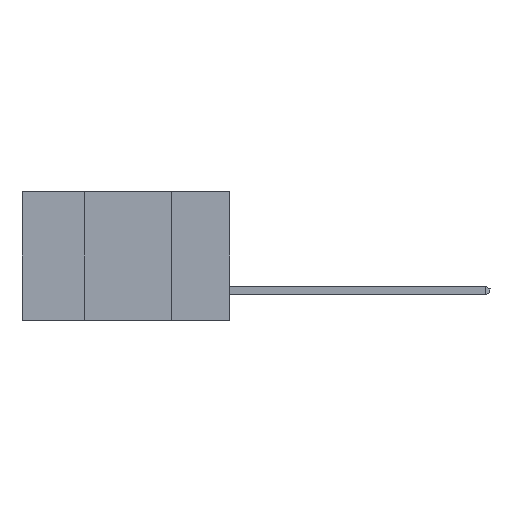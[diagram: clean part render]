
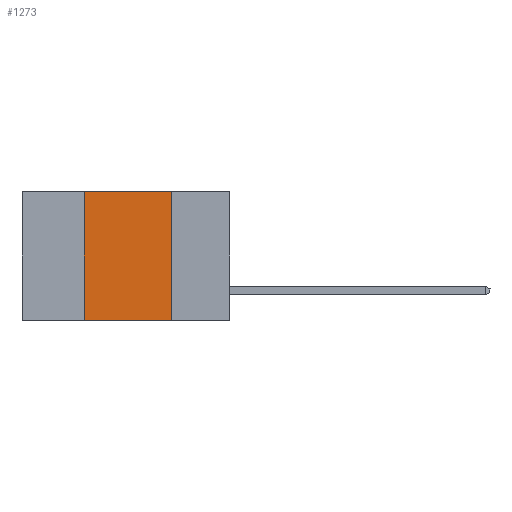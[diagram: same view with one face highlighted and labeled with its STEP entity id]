
A CAD part, left-side view. The second image highlights one B-rep face of the part: STEP entity #1273.
In plain terms, the highlighted planar face has unit normal (-1, 0, 0).
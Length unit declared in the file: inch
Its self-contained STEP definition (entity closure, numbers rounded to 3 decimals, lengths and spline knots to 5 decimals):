
#1056 = LINE ( 'NONE', #21196, #12962 ) ;
#1273 = ADVANCED_FACE ( 'NONE', ( #19097 ), #19217, .F. ) ;
#4416 = CARTESIAN_POINT ( 'NONE',  ( 0., 0.42, -0.37 ) ) ;
#5371 = LINE ( 'NONE', #20306, #11409 ) ;
#5848 = CARTESIAN_POINT ( 'NONE',  ( 0., 0.17, -0.37 ) ) ;
#5933 = ORIENTED_EDGE ( 'NONE', *, *, #13939, .F. ) ;
#7019 = CARTESIAN_POINT ( 'NONE',  ( 0., 0.42, 0. ) ) ;
#7093 = EDGE_CURVE ( 'NONE', #15746, #19948, #12179, .T. ) ;
#7341 = CARTESIAN_POINT ( 'NONE',  ( 0., 0.17, -0.37 ) ) ;
#7722 = EDGE_CURVE ( 'NONE', #10394, #15746, #1056, .T. ) ;
#9621 = DIRECTION ( 'NONE',  ( 1., 0., 0. ) ) ;
#10373 = DIRECTION ( 'NONE',  ( 0., 0., 1. ) ) ;
#10394 = VERTEX_POINT ( 'NONE', #7019 ) ;
#11375 = EDGE_LOOP ( 'NONE', ( #21436, #14454, #5933, #13914 ) ) ;
#11409 = VECTOR ( 'NONE', #10373, 39.37008 ) ;
#12171 = CARTESIAN_POINT ( 'NONE',  ( 0., 0.6, -0.37 ) ) ;
#12179 = LINE ( 'NONE', #5848, #17118 ) ;
#12962 = VECTOR ( 'NONE', #19569, 39.37008 ) ;
#13447 = CARTESIAN_POINT ( 'NONE',  ( 0., 0.17, 0. ) ) ;
#13914 = ORIENTED_EDGE ( 'NONE', *, *, #19448, .T. ) ;
#13939 = EDGE_CURVE ( 'NONE', #15495, #10394, #5371, .T. ) ;
#14454 = ORIENTED_EDGE ( 'NONE', *, *, #7722, .F. ) ;
#15495 = VERTEX_POINT ( 'NONE', #4416 ) ;
#15746 = VERTEX_POINT ( 'NONE', #13447 ) ;
#15823 = DIRECTION ( 'NONE',  ( 0., 0., -1. ) ) ;
#16032 = VECTOR ( 'NONE', #18819, 39.37008 ) ;
#17118 = VECTOR ( 'NONE', #17188, 39.37008 ) ;
#17188 = DIRECTION ( 'NONE',  ( 0., 0., -1. ) ) ;
#17677 = CARTESIAN_POINT ( 'NONE',  ( 0., 0.6, 0. ) ) ;
#18819 = DIRECTION ( 'NONE',  ( 0., -1., 0. ) ) ;
#19097 = FACE_OUTER_BOUND ( 'NONE', #11375, .T. ) ;
#19217 = PLANE ( 'NONE',  #19893 ) ;
#19448 = EDGE_CURVE ( 'NONE', #15495, #19948, #20048, .T. ) ;
#19569 = DIRECTION ( 'NONE',  ( 0., -1., 0. ) ) ;
#19893 = AXIS2_PLACEMENT_3D ( 'NONE', #17677, #9621, #15823 ) ;
#19948 = VERTEX_POINT ( 'NONE', #7341 ) ;
#20048 = LINE ( 'NONE', #12171, #16032 ) ;
#20306 = CARTESIAN_POINT ( 'NONE',  ( 0., 0.42, -0.37 ) ) ;
#21196 = CARTESIAN_POINT ( 'NONE',  ( 0., 0.6, 0. ) ) ;
#21436 = ORIENTED_EDGE ( 'NONE', *, *, #7093, .F. ) ;
